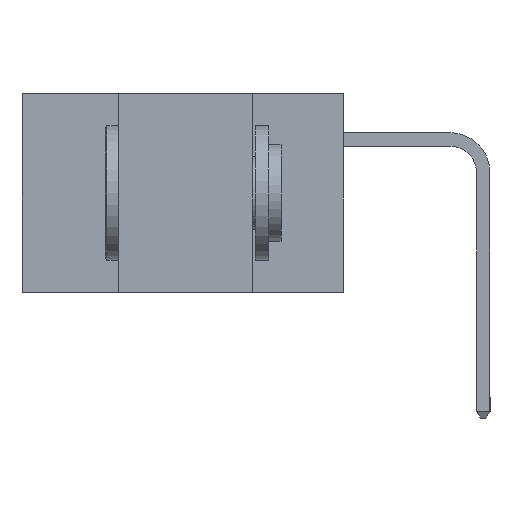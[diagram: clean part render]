
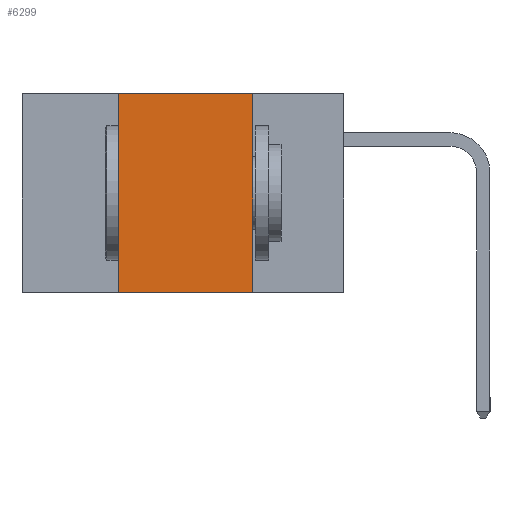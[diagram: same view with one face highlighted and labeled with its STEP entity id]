
A CAD part, left-side view. The second image highlights one B-rep face of the part: STEP entity #6299.
In plain terms, the highlighted planar face has unit normal (-1, 0, 0).
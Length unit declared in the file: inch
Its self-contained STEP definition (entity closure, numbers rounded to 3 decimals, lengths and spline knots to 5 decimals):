
#904 = CARTESIAN_POINT ( 'NONE',  ( 0., 0.42, -0.37 ) ) ;
#1449 = VECTOR ( 'NONE', #8268, 39.37008 ) ;
#2097 = VECTOR ( 'NONE', #17588, 39.37008 ) ;
#2388 = EDGE_CURVE ( 'NONE', #14843, #14411, #11942, .T. ) ;
#3483 = ORIENTED_EDGE ( 'NONE', *, *, #17692, .T. ) ;
#3637 = CARTESIAN_POINT ( 'NONE',  ( 0., 0.17, -0.37 ) ) ;
#3893 = LINE ( 'NONE', #17997, #23376 ) ;
#4604 = EDGE_LOOP ( 'NONE', ( #7239, #17085, #22449, #3483 ) ) ;
#4821 = EDGE_CURVE ( 'NONE', #14411, #4872, #6296, .T. ) ;
#4872 = VERTEX_POINT ( 'NONE', #10493 ) ;
#5070 = DIRECTION ( 'NONE',  ( 0., 0., 1. ) ) ;
#6296 = LINE ( 'NONE', #3637, #1449 ) ;
#6299 = ADVANCED_FACE ( 'NONE', ( #20677 ), #11815, .F. ) ;
#7239 = ORIENTED_EDGE ( 'NONE', *, *, #4821, .F. ) ;
#8147 = DIRECTION ( 'NONE',  ( 0., -1., 0. ) ) ;
#8268 = DIRECTION ( 'NONE',  ( 0., 0., -1. ) ) ;
#10493 = CARTESIAN_POINT ( 'NONE',  ( 0., 0.17, -0.37 ) ) ;
#10876 = DIRECTION ( 'NONE',  ( 0., 0., -1. ) ) ;
#11084 = DIRECTION ( 'NONE',  ( 1., 0., 0. ) ) ;
#11459 = CARTESIAN_POINT ( 'NONE',  ( 0., 0.17, 0. ) ) ;
#11698 = CARTESIAN_POINT ( 'NONE',  ( 0., 0.6, 0. ) ) ;
#11815 = PLANE ( 'NONE',  #21583 ) ;
#11942 = LINE ( 'NONE', #15030, #2097 ) ;
#12056 = VERTEX_POINT ( 'NONE', #904 ) ;
#14411 = VERTEX_POINT ( 'NONE', #11459 ) ;
#14843 = VERTEX_POINT ( 'NONE', #23539 ) ;
#15030 = CARTESIAN_POINT ( 'NONE',  ( 0., 0.6, 0. ) ) ;
#17085 = ORIENTED_EDGE ( 'NONE', *, *, #2388, .F. ) ;
#17588 = DIRECTION ( 'NONE',  ( 0., -1., 0. ) ) ;
#17692 = EDGE_CURVE ( 'NONE', #12056, #4872, #19366, .T. ) ;
#17997 = CARTESIAN_POINT ( 'NONE',  ( 0., 0.42, -0.37 ) ) ;
#19366 = LINE ( 'NONE', #22844, #20484 ) ;
#20484 = VECTOR ( 'NONE', #8147, 39.37008 ) ;
#20677 = FACE_OUTER_BOUND ( 'NONE', #4604, .T. ) ;
#21336 = EDGE_CURVE ( 'NONE', #12056, #14843, #3893, .T. ) ;
#21583 = AXIS2_PLACEMENT_3D ( 'NONE', #11698, #11084, #10876 ) ;
#22449 = ORIENTED_EDGE ( 'NONE', *, *, #21336, .F. ) ;
#22844 = CARTESIAN_POINT ( 'NONE',  ( 0., 0.6, -0.37 ) ) ;
#23376 = VECTOR ( 'NONE', #5070, 39.37008 ) ;
#23539 = CARTESIAN_POINT ( 'NONE',  ( 0., 0.42, 0. ) ) ;
